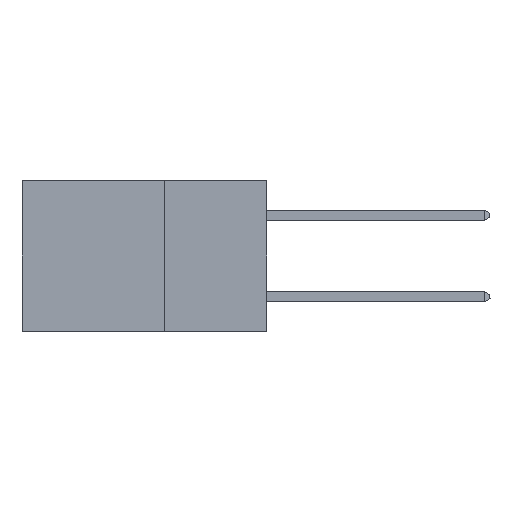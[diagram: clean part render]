
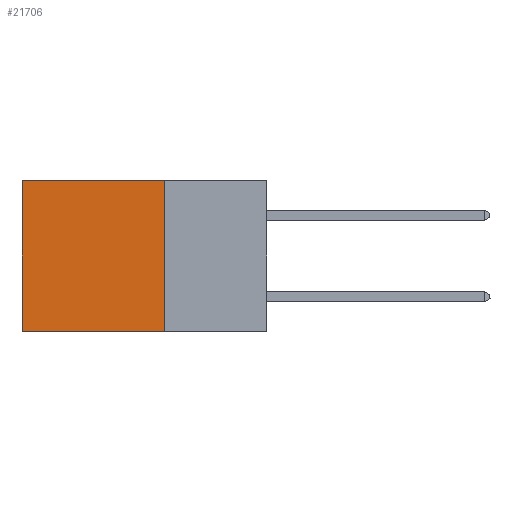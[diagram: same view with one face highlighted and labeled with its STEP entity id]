
A CAD part, left-side view. The second image highlights one B-rep face of the part: STEP entity #21706.
In plain terms, the highlighted planar face has unit normal (-1, 0, 0).
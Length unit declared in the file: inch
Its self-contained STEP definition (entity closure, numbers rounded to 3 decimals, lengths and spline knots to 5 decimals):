
#192 = VECTOR ( 'NONE', #23703, 39.37008 ) ;
#1821 = ORIENTED_EDGE ( 'NONE', *, *, #2075, .T. ) ;
#2075 = EDGE_CURVE ( 'NONE', #11643, #18287, #26278, .T. ) ;
#2286 = EDGE_CURVE ( 'NONE', #13112, #26867, #16827, .T. ) ;
#2476 = CARTESIAN_POINT ( 'NONE',  ( 0.2875, 0.6, 0. ) ) ;
#2885 = VECTOR ( 'NONE', #20046, 39.37008 ) ;
#4531 = EDGE_CURVE ( 'NONE', #26867, #18287, #15599, .T. ) ;
#4792 = LINE ( 'NONE', #23833, #7589 ) ;
#6520 = CARTESIAN_POINT ( 'NONE',  ( 0.2875, 0.25, 0. ) ) ;
#6925 = EDGE_CURVE ( 'NONE', #13112, #11643, #4792, .T. ) ;
#7589 = VECTOR ( 'NONE', #10442, 39.37008 ) ;
#8404 = CARTESIAN_POINT ( 'NONE',  ( 0.2875, 0.25, 0. ) ) ;
#8597 = DIRECTION ( 'NONE',  ( 0., 0., -1. ) ) ;
#9534 = DIRECTION ( 'NONE',  ( 0., 0., -1. ) ) ;
#10442 = DIRECTION ( 'NONE',  ( 0., 1., 0. ) ) ;
#10995 = CARTESIAN_POINT ( 'NONE',  ( 0.2875, 0.25, -0.37 ) ) ;
#11620 = CARTESIAN_POINT ( 'NONE',  ( 0.2875, 0.6, 0. ) ) ;
#11643 = VERTEX_POINT ( 'NONE', #2476 ) ;
#11882 = VECTOR ( 'NONE', #9534, 39.37008 ) ;
#12430 = FACE_OUTER_BOUND ( 'NONE', #19555, .T. ) ;
#13112 = VERTEX_POINT ( 'NONE', #6520 ) ;
#15599 = LINE ( 'NONE', #10995, #2885 ) ;
#16827 = LINE ( 'NONE', #16831, #192 ) ;
#16831 = CARTESIAN_POINT ( 'NONE',  ( 0.2875, 0.25, 0. ) ) ;
#17465 = DIRECTION ( 'NONE',  ( 1., 0., 0. ) ) ;
#18287 = VERTEX_POINT ( 'NONE', #19532 ) ;
#19532 = CARTESIAN_POINT ( 'NONE',  ( 0.2875, 0.6, -0.37 ) ) ;
#19555 = EDGE_LOOP ( 'NONE', ( #1821, #25355, #20132, #28788 ) ) ;
#20046 = DIRECTION ( 'NONE',  ( 0., 1., 0. ) ) ;
#20132 = ORIENTED_EDGE ( 'NONE', *, *, #2286, .F. ) ;
#21706 = ADVANCED_FACE ( 'NONE', ( #12430 ), #24440, .F. ) ;
#22708 = CARTESIAN_POINT ( 'NONE',  ( 0.2875, 0.25, -0.37 ) ) ;
#23703 = DIRECTION ( 'NONE',  ( 0., 0., -1. ) ) ;
#23833 = CARTESIAN_POINT ( 'NONE',  ( 0.2875, 0.25, 0. ) ) ;
#24440 = PLANE ( 'NONE',  #24448 ) ;
#24448 = AXIS2_PLACEMENT_3D ( 'NONE', #8404, #17465, #8597 ) ;
#25355 = ORIENTED_EDGE ( 'NONE', *, *, #4531, .F. ) ;
#26278 = LINE ( 'NONE', #11620, #11882 ) ;
#26867 = VERTEX_POINT ( 'NONE', #22708 ) ;
#28788 = ORIENTED_EDGE ( 'NONE', *, *, #6925, .T. ) ;
